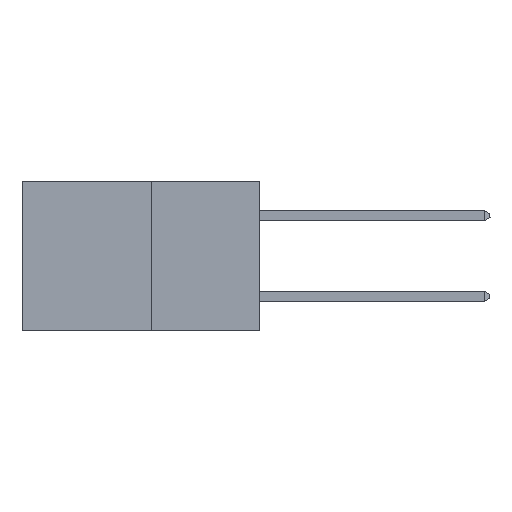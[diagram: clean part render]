
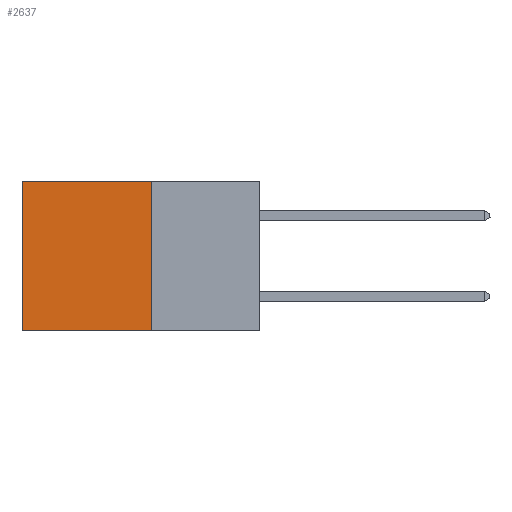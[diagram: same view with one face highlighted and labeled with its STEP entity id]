
A CAD part, left-side view. The second image highlights one B-rep face of the part: STEP entity #2637.
In plain terms, the highlighted planar face has unit normal (-1, 0, 0).
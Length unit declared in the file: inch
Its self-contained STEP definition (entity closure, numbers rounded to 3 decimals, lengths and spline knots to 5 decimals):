
#1663 = EDGE_CURVE ( 'NONE', #23658, #8276, #8531, .T. ) ;
#1767 = CARTESIAN_POINT ( 'NONE',  ( 0.277, 0.27, -0.37 ) ) ;
#2637 = ADVANCED_FACE ( 'NONE', ( #25872 ), #9569, .F. ) ;
#2951 = LINE ( 'NONE', #11141, #22067 ) ;
#3350 = VERTEX_POINT ( 'NONE', #27531 ) ;
#3875 = CARTESIAN_POINT ( 'NONE',  ( 0.277, 0.59, -0.37 ) ) ;
#4507 = CARTESIAN_POINT ( 'NONE',  ( 0.277, 0.27, -0.37 ) ) ;
#5111 = AXIS2_PLACEMENT_3D ( 'NONE', #23682, #16422, #15315 ) ;
#8276 = VERTEX_POINT ( 'NONE', #1767 ) ;
#8531 = LINE ( 'NONE', #4507, #21011 ) ;
#9505 = CARTESIAN_POINT ( 'NONE',  ( 0.277, 0.27, -0.37 ) ) ;
#9569 = PLANE ( 'NONE',  #5111 ) ;
#9652 = CARTESIAN_POINT ( 'NONE',  ( 0.277, 0.27, 0. ) ) ;
#10273 = VERTEX_POINT ( 'NONE', #13742 ) ;
#11141 = CARTESIAN_POINT ( 'NONE',  ( 0.277, 0.27, 0. ) ) ;
#11836 = VECTOR ( 'NONE', #23785, 39.37008 ) ;
#12028 = DIRECTION ( 'NONE',  ( 0., 1., 0. ) ) ;
#12387 = DIRECTION ( 'NONE',  ( 0., 0., -1. ) ) ;
#12615 = LINE ( 'NONE', #3875, #11836 ) ;
#13742 = CARTESIAN_POINT ( 'NONE',  ( 0.277, 0.59, -0.37 ) ) ;
#13969 = EDGE_CURVE ( 'NONE', #3350, #10273, #12615, .T. ) ;
#15315 = DIRECTION ( 'NONE',  ( 0., 0., -1. ) ) ;
#15513 = ORIENTED_EDGE ( 'NONE', *, *, #22669, .T. ) ;
#15848 = ORIENTED_EDGE ( 'NONE', *, *, #17975, .F. ) ;
#16422 = DIRECTION ( 'NONE',  ( 1., 0., 0. ) ) ;
#16625 = EDGE_LOOP ( 'NONE', ( #21651, #15848, #21969, #15513 ) ) ;
#17975 = EDGE_CURVE ( 'NONE', #8276, #10273, #18896, .T. ) ;
#18896 = LINE ( 'NONE', #9505, #31086 ) ;
#21011 = VECTOR ( 'NONE', #12387, 39.37008 ) ;
#21651 = ORIENTED_EDGE ( 'NONE', *, *, #13969, .T. ) ;
#21969 = ORIENTED_EDGE ( 'NONE', *, *, #1663, .F. ) ;
#22067 = VECTOR ( 'NONE', #25900, 39.37008 ) ;
#22669 = EDGE_CURVE ( 'NONE', #23658, #3350, #2951, .T. ) ;
#23658 = VERTEX_POINT ( 'NONE', #9652 ) ;
#23682 = CARTESIAN_POINT ( 'NONE',  ( 0.277, 0.27, -0.37 ) ) ;
#23785 = DIRECTION ( 'NONE',  ( 0., 0., -1. ) ) ;
#25872 = FACE_OUTER_BOUND ( 'NONE', #16625, .T. ) ;
#25900 = DIRECTION ( 'NONE',  ( 0., 1., 0. ) ) ;
#27531 = CARTESIAN_POINT ( 'NONE',  ( 0.277, 0.59, 0. ) ) ;
#31086 = VECTOR ( 'NONE', #12028, 39.37008 ) ;
